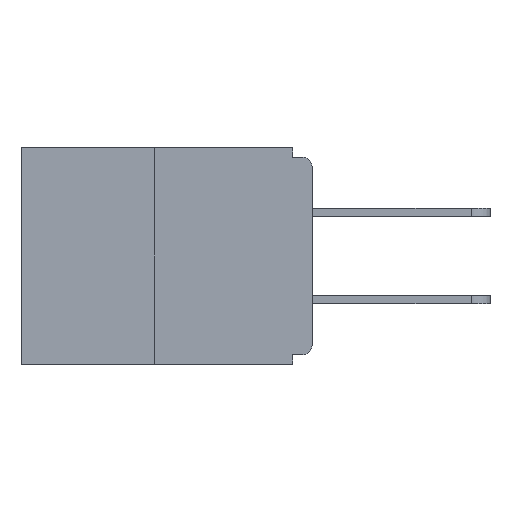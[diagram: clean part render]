
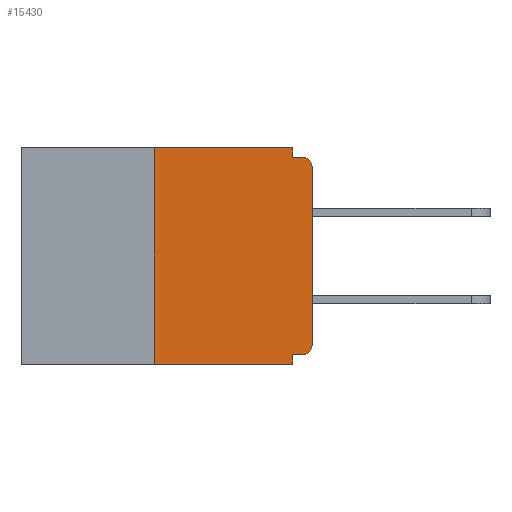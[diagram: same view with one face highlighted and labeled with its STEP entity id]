
A CAD part, left-side view. The second image highlights one B-rep face of the part: STEP entity #15430.
In plain terms, the highlighted planar face has unit normal (-1, 0, 0).
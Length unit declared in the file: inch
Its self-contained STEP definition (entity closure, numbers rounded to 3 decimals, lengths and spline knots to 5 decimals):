
#403 = CARTESIAN_POINT ( 'NONE',  ( 0., 0.25, 0. ) ) ;
#768 = VERTEX_POINT ( 'NONE', #3160 ) ;
#1677 = VECTOR ( 'NONE', #7945, 39.37008 ) ;
#3136 = ORIENTED_EDGE ( 'NONE', *, *, #7006, .T. ) ;
#3160 = CARTESIAN_POINT ( 'NONE',  ( 0., 0.031, 0. ) ) ;
#3229 = LINE ( 'NONE', #18740, #11505 ) ;
#3339 = DIRECTION ( 'NONE',  ( 0., 0., -1. ) ) ;
#4110 = ORIENTED_EDGE ( 'NONE', *, *, #13919, .F. ) ;
#4301 = ORIENTED_EDGE ( 'NONE', *, *, #22776, .F. ) ;
#4381 = CARTESIAN_POINT ( 'NONE',  ( 0., 0.031, -0.343 ) ) ;
#4383 = DIRECTION ( 'NONE',  ( 0., 1., 0. ) ) ;
#4891 = ORIENTED_EDGE ( 'NONE', *, *, #13471, .T. ) ;
#4966 = DIRECTION ( 'NONE',  ( 0., 0., -1. ) ) ;
#5480 = CARTESIAN_POINT ( 'NONE',  ( 0., 0.015, -0.015 ) ) ;
#5753 = DIRECTION ( 'NONE',  ( 0., 0., 1. ) ) ;
#5852 = VECTOR ( 'NONE', #13980, 39.37008 ) ;
#5870 = VERTEX_POINT ( 'NONE', #5480 ) ;
#5891 = VERTEX_POINT ( 'NONE', #15350 ) ;
#6073 = CARTESIAN_POINT ( 'NONE',  ( 0., 0., -0.313 ) ) ;
#6506 = CIRCLE ( 'NONE', #21464, 0.015 ) ;
#6712 = FACE_OUTER_BOUND ( 'NONE', #18293, .T. ) ;
#7006 = EDGE_CURVE ( 'NONE', #15564, #11565, #3229, .T. ) ;
#7137 = CARTESIAN_POINT ( 'NONE',  ( 0., 0.031, -0.343 ) ) ;
#7257 = DIRECTION ( 'NONE',  ( -1., 0., 0. ) ) ;
#7583 = VECTOR ( 'NONE', #9455, 39.37008 ) ;
#7833 = EDGE_CURVE ( 'NONE', #15564, #21674, #12657, .T. ) ;
#7945 = DIRECTION ( 'NONE',  ( 0., 0., -1. ) ) ;
#8521 = VERTEX_POINT ( 'NONE', #15861 ) ;
#8591 = DIRECTION ( 'NONE',  ( 0., 0., -1. ) ) ;
#8659 = EDGE_CURVE ( 'NONE', #10499, #10861, #8743, .T. ) ;
#8743 = LINE ( 'NONE', #20937, #21847 ) ;
#8910 = DIRECTION ( 'NONE',  ( 0., -1., 0. ) ) ;
#9054 = VERTEX_POINT ( 'NONE', #10557 ) ;
#9455 = DIRECTION ( 'NONE',  ( 0., -1., 0. ) ) ;
#9633 = VECTOR ( 'NONE', #4383, 39.37008 ) ;
#10499 = VERTEX_POINT ( 'NONE', #6073 ) ;
#10547 = ORIENTED_EDGE ( 'NONE', *, *, #21683, .F. ) ;
#10557 = CARTESIAN_POINT ( 'NONE',  ( 0., 0.031, -0.015 ) ) ;
#10861 = VERTEX_POINT ( 'NONE', #19502 ) ;
#11068 = DIRECTION ( 'NONE',  ( 0., 0., -1. ) ) ;
#11505 = VECTOR ( 'NONE', #14835, 39.37008 ) ;
#11565 = VERTEX_POINT ( 'NONE', #4381 ) ;
#11650 = ORIENTED_EDGE ( 'NONE', *, *, #15742, .F. ) ;
#12435 = DIRECTION ( 'NONE',  ( -1., 0., 0. ) ) ;
#12622 = LINE ( 'NONE', #15243, #7583 ) ;
#12657 = LINE ( 'NONE', #403, #5852 ) ;
#13471 = EDGE_CURVE ( 'NONE', #10861, #5870, #6506, .T. ) ;
#13664 = CARTESIAN_POINT ( 'NONE',  ( 0., 0., -0.328 ) ) ;
#13919 = EDGE_CURVE ( 'NONE', #9054, #5870, #18965, .T. ) ;
#13980 = DIRECTION ( 'NONE',  ( 0., 0., 1. ) ) ;
#14187 = LINE ( 'NONE', #7137, #21049 ) ;
#14594 = DIRECTION ( 'NONE',  ( 1., 0., 0. ) ) ;
#14828 = EDGE_CURVE ( 'NONE', #8521, #10499, #17756, .T. ) ;
#14835 = DIRECTION ( 'NONE',  ( 0., -1., 0. ) ) ;
#15243 = CARTESIAN_POINT ( 'NONE',  ( 0., 0.46, 0. ) ) ;
#15350 = CARTESIAN_POINT ( 'NONE',  ( 0., 0.031, -0.328 ) ) ;
#15430 = ADVANCED_FACE ( 'NONE', ( #6712 ), #16363, .F. ) ;
#15564 = VERTEX_POINT ( 'NONE', #20279 ) ;
#15742 = EDGE_CURVE ( 'NONE', #21674, #768, #12622, .T. ) ;
#15861 = CARTESIAN_POINT ( 'NONE',  ( 0., 0.015, -0.328 ) ) ;
#16363 = PLANE ( 'NONE',  #16912 ) ;
#16912 = AXIS2_PLACEMENT_3D ( 'NONE', #20236, #14594, #8591 ) ;
#17606 = CARTESIAN_POINT ( 'NONE',  ( 0., 0.25, 0. ) ) ;
#17756 = CIRCLE ( 'NONE', #22253, 0.015 ) ;
#18009 = LINE ( 'NONE', #22756, #1677 ) ;
#18293 = EDGE_LOOP ( 'NONE', ( #11650, #23595, #3136, #4301, #10547, #22450, #24361, #4891, #4110, #22525 ) ) ;
#18402 = VECTOR ( 'NONE', #8910, 39.37008 ) ;
#18740 = CARTESIAN_POINT ( 'NONE',  ( 0., 0.46, -0.343 ) ) ;
#18965 = LINE ( 'NONE', #20888, #18402 ) ;
#19502 = CARTESIAN_POINT ( 'NONE',  ( 0., 0., -0.03 ) ) ;
#20236 = CARTESIAN_POINT ( 'NONE',  ( 0., 0.46, 0. ) ) ;
#20279 = CARTESIAN_POINT ( 'NONE',  ( 0., 0.25, -0.343 ) ) ;
#20641 = CARTESIAN_POINT ( 'NONE',  ( 0., 0.015, -0.03 ) ) ;
#20888 = CARTESIAN_POINT ( 'NONE',  ( 0., 0., -0.015 ) ) ;
#20937 = CARTESIAN_POINT ( 'NONE',  ( 0., 0., 0. ) ) ;
#21049 = VECTOR ( 'NONE', #3339, 39.37008 ) ;
#21464 = AXIS2_PLACEMENT_3D ( 'NONE', #20641, #7257, #11068 ) ;
#21674 = VERTEX_POINT ( 'NONE', #17606 ) ;
#21683 = EDGE_CURVE ( 'NONE', #8521, #5891, #21802, .T. ) ;
#21802 = LINE ( 'NONE', #13664, #9633 ) ;
#21821 = CARTESIAN_POINT ( 'NONE',  ( 0., 0.015, -0.313 ) ) ;
#21847 = VECTOR ( 'NONE', #5753, 39.37008 ) ;
#22253 = AXIS2_PLACEMENT_3D ( 'NONE', #21821, #12435, #4966 ) ;
#22450 = ORIENTED_EDGE ( 'NONE', *, *, #14828, .T. ) ;
#22525 = ORIENTED_EDGE ( 'NONE', *, *, #23895, .F. ) ;
#22756 = CARTESIAN_POINT ( 'NONE',  ( 0., 0.031, 0. ) ) ;
#22776 = EDGE_CURVE ( 'NONE', #5891, #11565, #14187, .T. ) ;
#23595 = ORIENTED_EDGE ( 'NONE', *, *, #7833, .F. ) ;
#23895 = EDGE_CURVE ( 'NONE', #768, #9054, #18009, .T. ) ;
#24361 = ORIENTED_EDGE ( 'NONE', *, *, #8659, .T. ) ;
